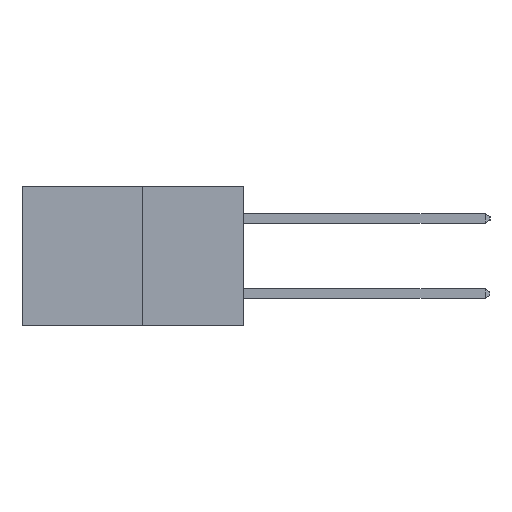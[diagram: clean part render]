
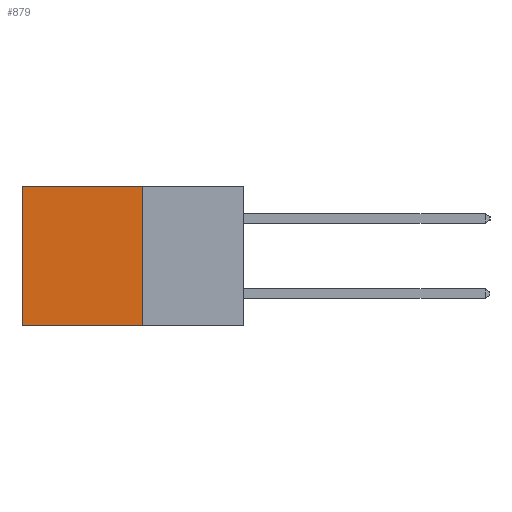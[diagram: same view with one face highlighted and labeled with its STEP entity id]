
A CAD part, left-side view. The second image highlights one B-rep face of the part: STEP entity #879.
In plain terms, the highlighted planar face has unit normal (-1, 0, 0).
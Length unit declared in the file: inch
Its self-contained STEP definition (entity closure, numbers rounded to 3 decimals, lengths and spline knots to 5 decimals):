
#879 = ADVANCED_FACE ( 'NONE', ( #22286 ), #7111, .F. ) ;
#1232 = LINE ( 'NONE', #19075, #13450 ) ;
#2109 = VERTEX_POINT ( 'NONE', #4542 ) ;
#2619 = VERTEX_POINT ( 'NONE', #28084 ) ;
#3148 = CARTESIAN_POINT ( 'NONE',  ( 0.277, 0.27, -0.37 ) ) ;
#4542 = CARTESIAN_POINT ( 'NONE',  ( 0.277, 0.27, 0. ) ) ;
#5646 = DIRECTION ( 'NONE',  ( 0., 1., 0. ) ) ;
#6003 = LINE ( 'NONE', #28645, #30775 ) ;
#7111 = PLANE ( 'NONE',  #18982 ) ;
#7190 = ORIENTED_EDGE ( 'NONE', *, *, #25101, .F. ) ;
#10274 = VERTEX_POINT ( 'NONE', #16290 ) ;
#10356 = VECTOR ( 'NONE', #5646, 39.37008 ) ;
#11854 = EDGE_LOOP ( 'NONE', ( #16251, #7190, #13627, #18921 ) ) ;
#11895 = DIRECTION ( 'NONE',  ( 0., 0., -1. ) ) ;
#13450 = VECTOR ( 'NONE', #21552, 39.37008 ) ;
#13481 = VERTEX_POINT ( 'NONE', #20966 ) ;
#13627 = ORIENTED_EDGE ( 'NONE', *, *, #20797, .F. ) ;
#16251 = ORIENTED_EDGE ( 'NONE', *, *, #23227, .T. ) ;
#16290 = CARTESIAN_POINT ( 'NONE',  ( 0.277, 0.59, -0.37 ) ) ;
#17635 = VECTOR ( 'NONE', #25923, 39.37008 ) ;
#18472 = EDGE_CURVE ( 'NONE', #2109, #2619, #24083, .T. ) ;
#18921 = ORIENTED_EDGE ( 'NONE', *, *, #18472, .T. ) ;
#18982 = AXIS2_PLACEMENT_3D ( 'NONE', #26599, #21298, #29979 ) ;
#19075 = CARTESIAN_POINT ( 'NONE',  ( 0.277, 0.59, -0.37 ) ) ;
#20797 = EDGE_CURVE ( 'NONE', #2109, #13481, #6003, .T. ) ;
#20966 = CARTESIAN_POINT ( 'NONE',  ( 0.277, 0.27, -0.37 ) ) ;
#21298 = DIRECTION ( 'NONE',  ( 1., 0., 0. ) ) ;
#21552 = DIRECTION ( 'NONE',  ( 0., 0., -1. ) ) ;
#22286 = FACE_OUTER_BOUND ( 'NONE', #11854, .T. ) ;
#23227 = EDGE_CURVE ( 'NONE', #2619, #10274, #1232, .T. ) ;
#23541 = CARTESIAN_POINT ( 'NONE',  ( 0.277, 0.27, 0. ) ) ;
#24083 = LINE ( 'NONE', #23541, #17635 ) ;
#25101 = EDGE_CURVE ( 'NONE', #13481, #10274, #29466, .T. ) ;
#25923 = DIRECTION ( 'NONE',  ( 0., 1., 0. ) ) ;
#26599 = CARTESIAN_POINT ( 'NONE',  ( 0.277, 0.27, -0.37 ) ) ;
#28084 = CARTESIAN_POINT ( 'NONE',  ( 0.277, 0.59, 0. ) ) ;
#28645 = CARTESIAN_POINT ( 'NONE',  ( 0.277, 0.27, -0.37 ) ) ;
#29466 = LINE ( 'NONE', #3148, #10356 ) ;
#29979 = DIRECTION ( 'NONE',  ( 0., 0., -1. ) ) ;
#30775 = VECTOR ( 'NONE', #11895, 39.37008 ) ;
